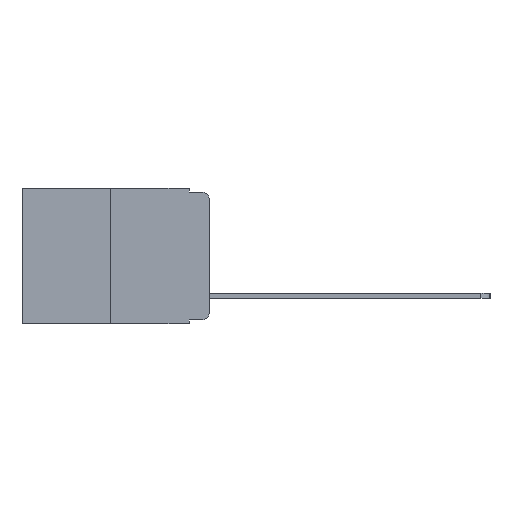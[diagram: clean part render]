
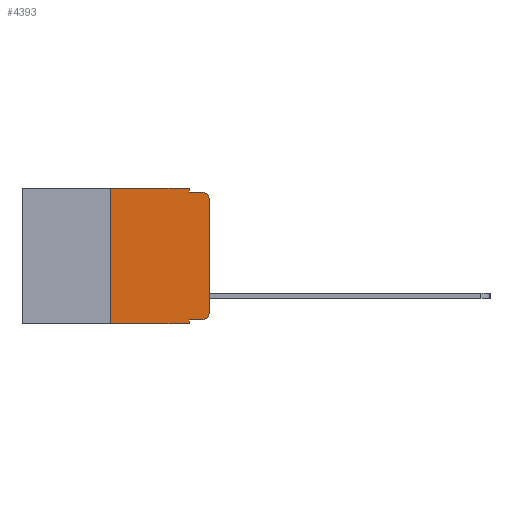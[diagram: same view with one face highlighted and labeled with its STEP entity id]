
A CAD part, left-side view. The second image highlights one B-rep face of the part: STEP entity #4393.
In plain terms, the highlighted planar face has unit normal (-1, 0, 0).
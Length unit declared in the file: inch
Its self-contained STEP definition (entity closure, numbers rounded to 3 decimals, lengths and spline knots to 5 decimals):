
#133 = ORIENTED_EDGE ( 'NONE', *, *, #3505, .F. ) ;
#249 = DIRECTION ( 'NONE',  ( 0., 0., -1. ) ) ;
#327 = VERTEX_POINT ( 'NONE', #3009 ) ;
#513 = CIRCLE ( 'NONE', #11759, 0.02 ) ;
#673 = CARTESIAN_POINT ( 'NONE',  ( 0., 0.473, 0. ) ) ;
#796 = ORIENTED_EDGE ( 'NONE', *, *, #6061, .T. ) ;
#1297 = LINE ( 'NONE', #5523, #11269 ) ;
#1635 = LINE ( 'NONE', #4788, #11256 ) ;
#1747 = CARTESIAN_POINT ( 'NONE',  ( 0., 0.02, -0.03 ) ) ;
#1898 = CARTESIAN_POINT ( 'NONE',  ( 0., 0., -0.03 ) ) ;
#1913 = CARTESIAN_POINT ( 'NONE',  ( 0., 0.02, -0.01 ) ) ;
#1946 = VERTEX_POINT ( 'NONE', #7334 ) ;
#2178 = VERTEX_POINT ( 'NONE', #1898 ) ;
#2210 = AXIS2_PLACEMENT_3D ( 'NONE', #1747, #8598, #2807 ) ;
#2223 = CARTESIAN_POINT ( 'NONE',  ( 0., 0.051, 0. ) ) ;
#2235 = LINE ( 'NONE', #673, #7151 ) ;
#2358 = VERTEX_POINT ( 'NONE', #7982 ) ;
#2654 = ORIENTED_EDGE ( 'NONE', *, *, #9210, .T. ) ;
#2807 = DIRECTION ( 'NONE',  ( 0., 0., -1. ) ) ;
#2953 = LINE ( 'NONE', #11295, #7806 ) ;
#3009 = CARTESIAN_POINT ( 'NONE',  ( 0., 0.051, -0.343 ) ) ;
#3505 = EDGE_CURVE ( 'NONE', #6182, #10838, #2235, .T. ) ;
#3590 = ORIENTED_EDGE ( 'NONE', *, *, #4730, .T. ) ;
#3738 = DIRECTION ( 'NONE',  ( 0., 0., -1. ) ) ;
#3829 = CIRCLE ( 'NONE', #2210, 0.02 ) ;
#3879 = DIRECTION ( 'NONE',  ( -1., 0., 0. ) ) ;
#3889 = CARTESIAN_POINT ( 'NONE',  ( 0., 0.473, -0.343 ) ) ;
#4011 = CARTESIAN_POINT ( 'NONE',  ( 0., 0.051, -0.01 ) ) ;
#4393 = ADVANCED_FACE ( 'NONE', ( #10758 ), #8208, .F. ) ;
#4676 = DIRECTION ( 'NONE',  ( 0., 0., -1. ) ) ;
#4730 = EDGE_CURVE ( 'NONE', #1946, #5071, #513, .T. ) ;
#4788 = CARTESIAN_POINT ( 'NONE',  ( 0., 0.25, 0. ) ) ;
#4890 = DIRECTION ( 'NONE',  ( 0., -1., 0. ) ) ;
#5071 = VERTEX_POINT ( 'NONE', #8192 ) ;
#5301 = ORIENTED_EDGE ( 'NONE', *, *, #8581, .F. ) ;
#5523 = CARTESIAN_POINT ( 'NONE',  ( 0., 0., 0. ) ) ;
#5616 = ORIENTED_EDGE ( 'NONE', *, *, #7312, .F. ) ;
#5785 = DIRECTION ( 'NONE',  ( 0., -1., 0. ) ) ;
#5858 = VECTOR ( 'NONE', #4890, 39.37008 ) ;
#5911 = ORIENTED_EDGE ( 'NONE', *, *, #12392, .T. ) ;
#6061 = EDGE_CURVE ( 'NONE', #2358, #1946, #7690, .T. ) ;
#6182 = VERTEX_POINT ( 'NONE', #6881 ) ;
#6316 = VECTOR ( 'NONE', #12161, 39.37008 ) ;
#6344 = DIRECTION ( 'NONE',  ( 1., 0., 0. ) ) ;
#6493 = LINE ( 'NONE', #12153, #8420 ) ;
#6622 = CARTESIAN_POINT ( 'NONE',  ( 0., 0.051, -0.01 ) ) ;
#6672 = EDGE_CURVE ( 'NONE', #2358, #327, #6493, .T. ) ;
#6714 = DIRECTION ( 'NONE',  ( 0., -1., 0. ) ) ;
#6881 = CARTESIAN_POINT ( 'NONE',  ( 0., 0.25, 0. ) ) ;
#7151 = VECTOR ( 'NONE', #5785, 39.37008 ) ;
#7255 = CARTESIAN_POINT ( 'NONE',  ( 0., 0.473, 0. ) ) ;
#7312 = EDGE_CURVE ( 'NONE', #9140, #6182, #1635, .T. ) ;
#7334 = CARTESIAN_POINT ( 'NONE',  ( 0., 0.02, -0.333 ) ) ;
#7690 = LINE ( 'NONE', #10425, #9877 ) ;
#7806 = VECTOR ( 'NONE', #3738, 39.37008 ) ;
#7821 = ORIENTED_EDGE ( 'NONE', *, *, #7938, .F. ) ;
#7938 = EDGE_CURVE ( 'NONE', #10838, #11321, #2953, .T. ) ;
#7982 = CARTESIAN_POINT ( 'NONE',  ( 0., 0.051, -0.333 ) ) ;
#8087 = VERTEX_POINT ( 'NONE', #1913 ) ;
#8192 = CARTESIAN_POINT ( 'NONE',  ( 0., 0., -0.313 ) ) ;
#8208 = PLANE ( 'NONE',  #10763 ) ;
#8420 = VECTOR ( 'NONE', #4676, 39.37008 ) ;
#8425 = ORIENTED_EDGE ( 'NONE', *, *, #6672, .F. ) ;
#8581 = EDGE_CURVE ( 'NONE', #11321, #8087, #8832, .T. ) ;
#8598 = DIRECTION ( 'NONE',  ( -1., 0., 0. ) ) ;
#8832 = LINE ( 'NONE', #6622, #6316 ) ;
#9140 = VERTEX_POINT ( 'NONE', #9428 ) ;
#9210 = EDGE_CURVE ( 'NONE', #2178, #8087, #3829, .T. ) ;
#9428 = CARTESIAN_POINT ( 'NONE',  ( 0., 0.25, -0.343 ) ) ;
#9622 = CARTESIAN_POINT ( 'NONE',  ( 0., 0.02, -0.313 ) ) ;
#9877 = VECTOR ( 'NONE', #6714, 39.37008 ) ;
#10422 = EDGE_CURVE ( 'NONE', #5071, #2178, #1297, .T. ) ;
#10425 = CARTESIAN_POINT ( 'NONE',  ( 0., 0.051, -0.333 ) ) ;
#10522 = DIRECTION ( 'NONE',  ( 0., 0., -1. ) ) ;
#10758 = FACE_OUTER_BOUND ( 'NONE', #11099, .T. ) ;
#10763 = AXIS2_PLACEMENT_3D ( 'NONE', #7255, #6344, #249 ) ;
#10800 = LINE ( 'NONE', #3889, #5858 ) ;
#10838 = VERTEX_POINT ( 'NONE', #2223 ) ;
#11091 = DIRECTION ( 'NONE',  ( 0., 0., 1. ) ) ;
#11099 = EDGE_LOOP ( 'NONE', ( #12407, #2654, #5301, #7821, #133, #5616, #5911, #8425, #796, #3590 ) ) ;
#11256 = VECTOR ( 'NONE', #12261, 39.37008 ) ;
#11269 = VECTOR ( 'NONE', #11091, 39.37008 ) ;
#11295 = CARTESIAN_POINT ( 'NONE',  ( 0., 0.051, 0. ) ) ;
#11321 = VERTEX_POINT ( 'NONE', #4011 ) ;
#11759 = AXIS2_PLACEMENT_3D ( 'NONE', #9622, #3879, #10522 ) ;
#12153 = CARTESIAN_POINT ( 'NONE',  ( 0., 0.051, 0. ) ) ;
#12161 = DIRECTION ( 'NONE',  ( 0., -1., 0. ) ) ;
#12261 = DIRECTION ( 'NONE',  ( 0., 0., 1. ) ) ;
#12392 = EDGE_CURVE ( 'NONE', #9140, #327, #10800, .T. ) ;
#12407 = ORIENTED_EDGE ( 'NONE', *, *, #10422, .T. ) ;
